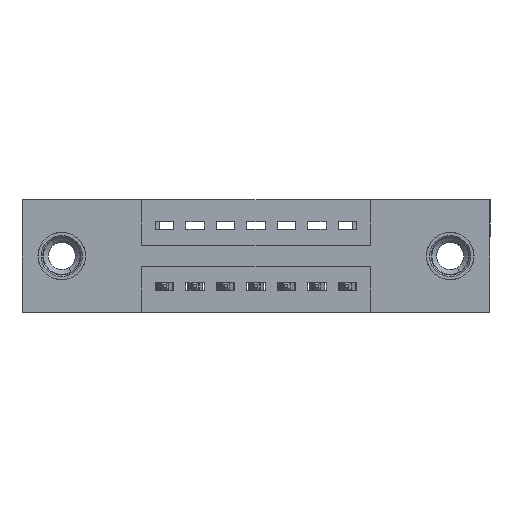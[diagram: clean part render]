
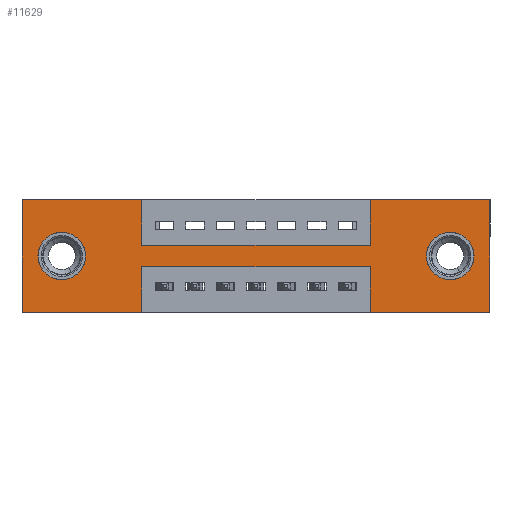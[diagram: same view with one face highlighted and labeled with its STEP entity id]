
A CAD part, front view. The second image highlights one B-rep face of the part: STEP entity #11629.
In plain terms, the highlighted planar face has unit normal (0, -1, 0).
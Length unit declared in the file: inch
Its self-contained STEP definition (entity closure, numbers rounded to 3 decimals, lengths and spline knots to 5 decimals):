
#18 = ORIENTED_EDGE ( 'NONE', *, *, #2343, .F. ) ;
#78 = CARTESIAN_POINT ( 'NONE',  ( 0.13, 0., -0.185 ) ) ;
#305 = LINE ( 'NONE', #8280, #4429 ) ;
#402 = CARTESIAN_POINT ( 'NONE',  ( 0.3925, 0., -0.22 ) ) ;
#417 = CIRCLE ( 'NONE', #5216, 0.078 ) ;
#443 = LINE ( 'NONE', #2685, #1177 ) ;
#664 = DIRECTION ( 'NONE',  ( -1., 0., 0. ) ) ;
#695 = CARTESIAN_POINT ( 'NONE',  ( 1.535, 0., 0. ) ) ;
#732 = FACE_OUTER_BOUND ( 'NONE', #11590, .T. ) ;
#806 = ORIENTED_EDGE ( 'NONE', *, *, #1207, .F. ) ;
#1000 = ORIENTED_EDGE ( 'NONE', *, *, #5738, .F. ) ;
#1177 = VECTOR ( 'NONE', #4545, 39.37008 ) ;
#1178 = DIRECTION ( 'NONE',  ( 0., 0., 1. ) ) ;
#1207 = EDGE_CURVE ( 'NONE', #2905, #4918, #6632, .T. ) ;
#1252 = CARTESIAN_POINT ( 'NONE',  ( 0., 0., -0.37 ) ) ;
#1441 = CARTESIAN_POINT ( 'NONE',  ( 1.535, 0., -0.37 ) ) ;
#1467 = CARTESIAN_POINT ( 'NONE',  ( 0.3925, 0., -0.15 ) ) ;
#1544 = DIRECTION ( 'NONE',  ( 0., 1., 0. ) ) ;
#1588 = CIRCLE ( 'NONE', #5424, 0.078 ) ;
#1713 = VECTOR ( 'NONE', #6656, 39.37008 ) ;
#1744 = CARTESIAN_POINT ( 'NONE',  ( 0., 0., 0. ) ) ;
#1880 = ORIENTED_EDGE ( 'NONE', *, *, #8019, .F. ) ;
#1918 = CIRCLE ( 'NONE', #4027, 0.078 ) ;
#1931 = LINE ( 'NONE', #402, #5596 ) ;
#2221 = PLANE ( 'NONE',  #11178 ) ;
#2293 = VERTEX_POINT ( 'NONE', #3349 ) ;
#2343 = EDGE_CURVE ( 'NONE', #8106, #6783, #4699, .T. ) ;
#2489 = EDGE_CURVE ( 'NONE', #10140, #12088, #1588, .T. ) ;
#2495 = ORIENTED_EDGE ( 'NONE', *, *, #12027, .F. ) ;
#2503 = VERTEX_POINT ( 'NONE', #4898 ) ;
#2662 = VECTOR ( 'NONE', #8429, 39.37008 ) ;
#2685 = CARTESIAN_POINT ( 'NONE',  ( 0., 0., 0. ) ) ;
#2705 = CARTESIAN_POINT ( 'NONE',  ( 0.13, 0., -0.107 ) ) ;
#2719 = DIRECTION ( 'NONE',  ( 0., -1., 0. ) ) ;
#2793 = LINE ( 'NONE', #6831, #7497 ) ;
#2809 = EDGE_CURVE ( 'NONE', #4918, #11535, #11153, .T. ) ;
#2839 = ORIENTED_EDGE ( 'NONE', *, *, #6519, .T. ) ;
#2905 = VERTEX_POINT ( 'NONE', #7860 ) ;
#2962 = DIRECTION ( 'NONE',  ( 0., 1., 0. ) ) ;
#3085 = CARTESIAN_POINT ( 'NONE',  ( 0., 0., -0.37 ) ) ;
#3194 = DIRECTION ( 'NONE',  ( 0., 0., -1. ) ) ;
#3326 = DIRECTION ( 'NONE',  ( 1., 0., 0. ) ) ;
#3349 = CARTESIAN_POINT ( 'NONE',  ( 1.1425, 0., 0. ) ) ;
#3367 = ORIENTED_EDGE ( 'NONE', *, *, #5721, .T. ) ;
#3477 = CARTESIAN_POINT ( 'NONE',  ( 0.13, 0., -0.185 ) ) ;
#3567 = DIRECTION ( 'NONE',  ( 0., 0., -1. ) ) ;
#3648 = CARTESIAN_POINT ( 'NONE',  ( 0.3925, 0., -0.37 ) ) ;
#3670 = DIRECTION ( 'NONE',  ( 1., 0., 0. ) ) ;
#4027 = AXIS2_PLACEMENT_3D ( 'NONE', #5054, #8829, #3194 ) ;
#4132 = VERTEX_POINT ( 'NONE', #5286 ) ;
#4314 = DIRECTION ( 'NONE',  ( 0., 1., 0. ) ) ;
#4407 = CARTESIAN_POINT ( 'NONE',  ( 0., 0., 0. ) ) ;
#4424 = VECTOR ( 'NONE', #664, 39.37008 ) ;
#4429 = VECTOR ( 'NONE', #3670, 39.37008 ) ;
#4545 = DIRECTION ( 'NONE',  ( 0., 0., 1. ) ) ;
#4699 = LINE ( 'NONE', #7399, #12176 ) ;
#4898 = CARTESIAN_POINT ( 'NONE',  ( 0.3925, 0., -0.22 ) ) ;
#4918 = VERTEX_POINT ( 'NONE', #9712 ) ;
#5002 = CARTESIAN_POINT ( 'NONE',  ( 1.1425, 0., -0.15 ) ) ;
#5054 = CARTESIAN_POINT ( 'NONE',  ( 1.405, 0., -0.185 ) ) ;
#5216 = AXIS2_PLACEMENT_3D ( 'NONE', #9907, #4314, #10889 ) ;
#5286 = CARTESIAN_POINT ( 'NONE',  ( 1.405, 0., -0.263 ) ) ;
#5411 = CARTESIAN_POINT ( 'NONE',  ( 0.13, 0., -0.263 ) ) ;
#5424 = AXIS2_PLACEMENT_3D ( 'NONE', #78, #2962, #1178 ) ;
#5516 = EDGE_CURVE ( 'NONE', #11535, #8593, #305, .T. ) ;
#5519 = LINE ( 'NONE', #11552, #10357 ) ;
#5545 = DIRECTION ( 'NONE',  ( 0., 0., -1. ) ) ;
#5560 = EDGE_CURVE ( 'NONE', #8400, #2905, #443, .T. ) ;
#5596 = VECTOR ( 'NONE', #6149, 39.37008 ) ;
#5661 = CARTESIAN_POINT ( 'NONE',  ( 1.1425, 0., 0. ) ) ;
#5721 = EDGE_CURVE ( 'NONE', #4132, #5775, #1918, .T. ) ;
#5738 = EDGE_CURVE ( 'NONE', #6783, #8882, #2793, .T. ) ;
#5775 = VERTEX_POINT ( 'NONE', #8691 ) ;
#5810 = CIRCLE ( 'NONE', #9324, 0.078 ) ;
#5893 = VECTOR ( 'NONE', #3326, 39.37008 ) ;
#5979 = VECTOR ( 'NONE', #9986, 39.37008 ) ;
#6022 = ORIENTED_EDGE ( 'NONE', *, *, #5516, .F. ) ;
#6057 = ORIENTED_EDGE ( 'NONE', *, *, #2489, .T. ) ;
#6086 = ORIENTED_EDGE ( 'NONE', *, *, #2809, .F. ) ;
#6149 = DIRECTION ( 'NONE',  ( -1., 0., 0. ) ) ;
#6519 = EDGE_CURVE ( 'NONE', #5775, #4132, #417, .T. ) ;
#6632 = LINE ( 'NONE', #4407, #5893 ) ;
#6656 = DIRECTION ( 'NONE',  ( 0., 0., 1. ) ) ;
#6701 = ORIENTED_EDGE ( 'NONE', *, *, #11936, .F. ) ;
#6707 = VECTOR ( 'NONE', #3567, 39.37008 ) ;
#6783 = VERTEX_POINT ( 'NONE', #1441 ) ;
#6831 = CARTESIAN_POINT ( 'NONE',  ( 0., 0., -0.37 ) ) ;
#7192 = ORIENTED_EDGE ( 'NONE', *, *, #11593, .F. ) ;
#7223 = ORIENTED_EDGE ( 'NONE', *, *, #8509, .F. ) ;
#7337 = CARTESIAN_POINT ( 'NONE',  ( 1.1425, 0., -0.22 ) ) ;
#7399 = CARTESIAN_POINT ( 'NONE',  ( 1.535, 0., 0. ) ) ;
#7497 = VECTOR ( 'NONE', #7847, 39.37008 ) ;
#7526 = LINE ( 'NONE', #1744, #2662 ) ;
#7600 = LINE ( 'NONE', #5661, #1713 ) ;
#7847 = DIRECTION ( 'NONE',  ( -1., 0., 0. ) ) ;
#7860 = CARTESIAN_POINT ( 'NONE',  ( 0., 0., 0. ) ) ;
#7949 = EDGE_CURVE ( 'NONE', #12088, #10140, #5810, .T. ) ;
#8019 = EDGE_CURVE ( 'NONE', #2503, #8603, #9189, .T. ) ;
#8106 = VERTEX_POINT ( 'NONE', #695 ) ;
#8280 = CARTESIAN_POINT ( 'NONE',  ( 0.3925, 0., -0.15 ) ) ;
#8353 = EDGE_CURVE ( 'NONE', #8882, #10773, #5519, .T. ) ;
#8400 = VERTEX_POINT ( 'NONE', #1252 ) ;
#8429 = DIRECTION ( 'NONE',  ( 1., 0., 0. ) ) ;
#8509 = EDGE_CURVE ( 'NONE', #8593, #2293, #7600, .T. ) ;
#8593 = VERTEX_POINT ( 'NONE', #5002 ) ;
#8603 = VERTEX_POINT ( 'NONE', #8768 ) ;
#8691 = CARTESIAN_POINT ( 'NONE',  ( 1.405, 0., -0.107 ) ) ;
#8768 = CARTESIAN_POINT ( 'NONE',  ( 0.3925, 0., -0.37 ) ) ;
#8829 = DIRECTION ( 'NONE',  ( 0., 1., 0. ) ) ;
#8882 = VERTEX_POINT ( 'NONE', #10163 ) ;
#9042 = CARTESIAN_POINT ( 'NONE',  ( 0.3925, 0., 0. ) ) ;
#9189 = LINE ( 'NONE', #3648, #6707 ) ;
#9265 = EDGE_LOOP ( 'NONE', ( #6057, #11320 ) ) ;
#9324 = AXIS2_PLACEMENT_3D ( 'NONE', #3477, #1544, #11814 ) ;
#9712 = CARTESIAN_POINT ( 'NONE',  ( 0.3925, 0., 0. ) ) ;
#9907 = CARTESIAN_POINT ( 'NONE',  ( 1.405, 0., -0.185 ) ) ;
#9976 = LINE ( 'NONE', #11090, #4424 ) ;
#9986 = DIRECTION ( 'NONE',  ( 0., 0., -1. ) ) ;
#10140 = VERTEX_POINT ( 'NONE', #2705 ) ;
#10163 = CARTESIAN_POINT ( 'NONE',  ( 1.1425, 0., -0.37 ) ) ;
#10357 = VECTOR ( 'NONE', #10756, 39.37008 ) ;
#10431 = EDGE_LOOP ( 'NONE', ( #2839, #3367 ) ) ;
#10656 = DIRECTION ( 'NONE',  ( 0., 0., -1. ) ) ;
#10713 = ORIENTED_EDGE ( 'NONE', *, *, #8353, .F. ) ;
#10756 = DIRECTION ( 'NONE',  ( 0., 0., 1. ) ) ;
#10773 = VERTEX_POINT ( 'NONE', #7337 ) ;
#10889 = DIRECTION ( 'NONE',  ( 0., 0., -1. ) ) ;
#11090 = CARTESIAN_POINT ( 'NONE',  ( 0., 0., -0.37 ) ) ;
#11153 = LINE ( 'NONE', #9042, #5979 ) ;
#11178 = AXIS2_PLACEMENT_3D ( 'NONE', #3085, #2719, #10656 ) ;
#11320 = ORIENTED_EDGE ( 'NONE', *, *, #7949, .T. ) ;
#11430 = ORIENTED_EDGE ( 'NONE', *, *, #5560, .F. ) ;
#11535 = VERTEX_POINT ( 'NONE', #1467 ) ;
#11552 = CARTESIAN_POINT ( 'NONE',  ( 1.1425, 0., -0.37 ) ) ;
#11590 = EDGE_LOOP ( 'NONE', ( #1880, #6701, #10713, #1000, #18, #7192, #7223, #6022, #6086, #806, #11430, #2495 ) ) ;
#11593 = EDGE_CURVE ( 'NONE', #2293, #8106, #7526, .T. ) ;
#11625 = FACE_BOUND ( 'NONE', #10431, .T. ) ;
#11629 = ADVANCED_FACE ( 'NONE', ( #11625, #11914, #732 ), #2221, .T. ) ;
#11814 = DIRECTION ( 'NONE',  ( 0., 0., 1. ) ) ;
#11914 = FACE_BOUND ( 'NONE', #9265, .T. ) ;
#11936 = EDGE_CURVE ( 'NONE', #10773, #2503, #1931, .T. ) ;
#12027 = EDGE_CURVE ( 'NONE', #8603, #8400, #9976, .T. ) ;
#12088 = VERTEX_POINT ( 'NONE', #5411 ) ;
#12176 = VECTOR ( 'NONE', #5545, 39.37008 ) ;
